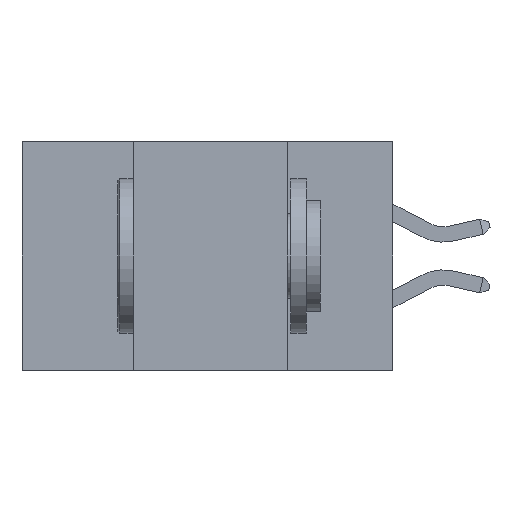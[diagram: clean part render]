
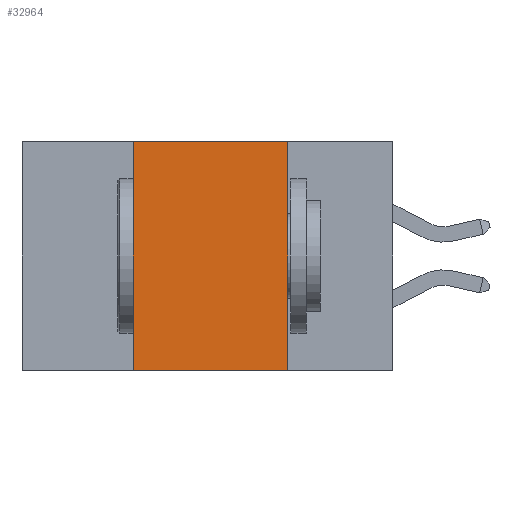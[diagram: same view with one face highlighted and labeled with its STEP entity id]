
A CAD part, left-side view. The second image highlights one B-rep face of the part: STEP entity #32964.
In plain terms, the highlighted planar face has unit normal (-1, 0, 0).
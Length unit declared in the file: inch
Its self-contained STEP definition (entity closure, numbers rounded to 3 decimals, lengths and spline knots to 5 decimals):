
#146 = ORIENTED_EDGE ( 'NONE', *, *, #16251, .F. ) ;
#2576 = EDGE_CURVE ( 'NONE', #19328, #24504, #37769, .T. ) ;
#2911 = DIRECTION ( 'NONE',  ( 0., 0., -1. ) ) ;
#3074 = DIRECTION ( 'NONE',  ( 0., -1., 0. ) ) ;
#4769 = EDGE_LOOP ( 'NONE', ( #146, #37918, #23450, #33890 ) ) ;
#7262 = EDGE_CURVE ( 'NONE', #11230, #29047, #10945, .T. ) ;
#7630 = CARTESIAN_POINT ( 'NONE',  ( 0., 0.17, 0. ) ) ;
#9071 = PLANE ( 'NONE',  #29715 ) ;
#9649 = CARTESIAN_POINT ( 'NONE',  ( 0., 0.42, 0. ) ) ;
#10945 = LINE ( 'NONE', #17345, #19652 ) ;
#11019 = DIRECTION ( 'NONE',  ( 0., 0., -1. ) ) ;
#11230 = VERTEX_POINT ( 'NONE', #12068 ) ;
#12068 = CARTESIAN_POINT ( 'NONE',  ( 0., 0.42, -0.37 ) ) ;
#13646 = CARTESIAN_POINT ( 'NONE',  ( 0., 0.17, -0.37 ) ) ;
#16251 = EDGE_CURVE ( 'NONE', #24504, #29047, #34878, .T. ) ;
#16721 = VECTOR ( 'NONE', #30498, 39.37008 ) ;
#17345 = CARTESIAN_POINT ( 'NONE',  ( 0., 0.6, -0.37 ) ) ;
#19328 = VERTEX_POINT ( 'NONE', #9649 ) ;
#19652 = VECTOR ( 'NONE', #23810, 39.37008 ) ;
#22027 = EDGE_CURVE ( 'NONE', #11230, #19328, #24929, .T. ) ;
#23450 = ORIENTED_EDGE ( 'NONE', *, *, #22027, .F. ) ;
#23810 = DIRECTION ( 'NONE',  ( 0., -1., 0. ) ) ;
#24457 = DIRECTION ( 'NONE',  ( 1., 0., 0. ) ) ;
#24504 = VERTEX_POINT ( 'NONE', #38034 ) ;
#24929 = LINE ( 'NONE', #36576, #16721 ) ;
#26699 = VECTOR ( 'NONE', #3074, 39.37008 ) ;
#27458 = CARTESIAN_POINT ( 'NONE',  ( 0., 0.6, 0. ) ) ;
#29047 = VERTEX_POINT ( 'NONE', #13646 ) ;
#29715 = AXIS2_PLACEMENT_3D ( 'NONE', #27458, #24457, #2911 ) ;
#30289 = FACE_OUTER_BOUND ( 'NONE', #4769, .T. ) ;
#30498 = DIRECTION ( 'NONE',  ( 0., 0., 1. ) ) ;
#32964 = ADVANCED_FACE ( 'NONE', ( #30289 ), #9071, .F. ) ;
#32989 = VECTOR ( 'NONE', #11019, 39.37008 ) ;
#33890 = ORIENTED_EDGE ( 'NONE', *, *, #7262, .T. ) ;
#34878 = LINE ( 'NONE', #7630, #32989 ) ;
#36576 = CARTESIAN_POINT ( 'NONE',  ( 0., 0.42, 0. ) ) ;
#37175 = CARTESIAN_POINT ( 'NONE',  ( 0., 0.6, 0. ) ) ;
#37769 = LINE ( 'NONE', #37175, #26699 ) ;
#37918 = ORIENTED_EDGE ( 'NONE', *, *, #2576, .F. ) ;
#38034 = CARTESIAN_POINT ( 'NONE',  ( 0., 0.17, 0. ) ) ;
